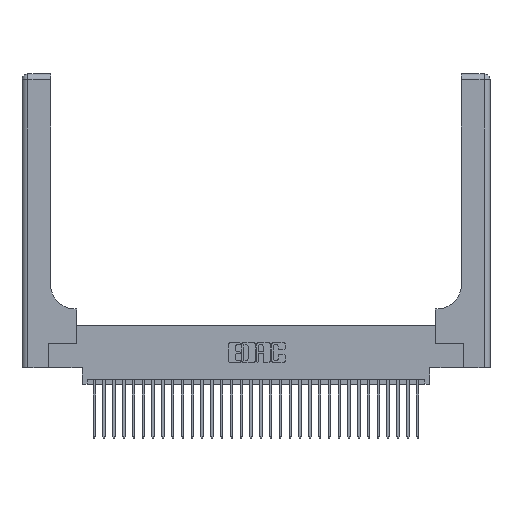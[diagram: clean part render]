
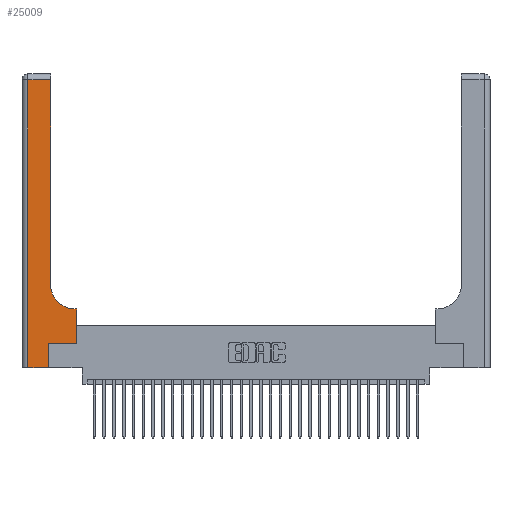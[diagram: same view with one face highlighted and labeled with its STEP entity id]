
A CAD part, top view. The second image highlights one B-rep face of the part: STEP entity #25009.
In plain terms, the highlighted planar face has unit normal (0, 0, 1).
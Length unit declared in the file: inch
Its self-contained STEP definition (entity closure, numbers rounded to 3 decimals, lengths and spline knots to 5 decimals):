
#437 = LINE ( 'NONE', #23626, #13341 ) ;
#452 = CARTESIAN_POINT ( 'NONE',  ( 0.2915, 3., 0.37 ) ) ;
#561 = CARTESIAN_POINT ( 'NONE',  ( 0.2915, 0.6, 0.37 ) ) ;
#865 = CARTESIAN_POINT ( 'NONE',  ( 0.2915, 2.94, 0.37 ) ) ;
#1384 = CARTESIAN_POINT ( 'NONE',  ( 0.269, 0., 0.37 ) ) ;
#1881 = VERTEX_POINT ( 'NONE', #16991 ) ;
#2483 = ORIENTED_EDGE ( 'NONE', *, *, #30789, .T. ) ;
#2496 = CARTESIAN_POINT ( 'NONE',  ( 0.2915, 0.85, 0.37 ) ) ;
#3045 = ORIENTED_EDGE ( 'NONE', *, *, #4793, .T. ) ;
#3761 = DIRECTION ( 'NONE',  ( 0., 1., 0. ) ) ;
#4261 = VECTOR ( 'NONE', #16527, 39.37008 ) ;
#4507 = AXIS2_PLACEMENT_3D ( 'NONE', #21239, #13704, #13822 ) ;
#4793 = EDGE_CURVE ( 'NONE', #21407, #13667, #21918, .T. ) ;
#5126 = LINE ( 'NONE', #13885, #5511 ) ;
#5150 = AXIS2_PLACEMENT_3D ( 'NONE', #10960, #29333, #16827 ) ;
#5359 = VERTEX_POINT ( 'NONE', #17052 ) ;
#5511 = VECTOR ( 'NONE', #26404, 39.37008 ) ;
#5769 = CARTESIAN_POINT ( 'NONE',  ( 0.5415, 0.6, 0.37 ) ) ;
#5824 = LINE ( 'NONE', #1384, #4261 ) ;
#6799 = EDGE_CURVE ( 'NONE', #12042, #1881, #5824, .T. ) ;
#7576 = LINE ( 'NONE', #21021, #11611 ) ;
#8176 = EDGE_CURVE ( 'NONE', #11689, #12443, #8550, .T. ) ;
#8550 = CIRCLE ( 'NONE', #4507, 0.25 ) ;
#9730 = CARTESIAN_POINT ( 'NONE',  ( 0.5585, 0.25, 0.37 ) ) ;
#9864 = ORIENTED_EDGE ( 'NONE', *, *, #23254, .T. ) ;
#10960 = CARTESIAN_POINT ( 'NONE',  ( 0., 3., 0.37 ) ) ;
#11039 = VERTEX_POINT ( 'NONE', #9730 ) ;
#11091 = FACE_OUTER_BOUND ( 'NONE', #13476, .T. ) ;
#11585 = CARTESIAN_POINT ( 'NONE',  ( 0.269, 0., 0.37 ) ) ;
#11611 = VECTOR ( 'NONE', #15913, 39.37008 ) ;
#11689 = VERTEX_POINT ( 'NONE', #5769 ) ;
#11744 = EDGE_CURVE ( 'NONE', #1881, #11039, #437, .T. ) ;
#11920 = LINE ( 'NONE', #22999, #21047 ) ;
#12042 = VERTEX_POINT ( 'NONE', #11585 ) ;
#12222 = LINE ( 'NONE', #452, #17028 ) ;
#12385 = VECTOR ( 'NONE', #31955, 39.37008 ) ;
#12443 = VERTEX_POINT ( 'NONE', #2496 ) ;
#13009 = ORIENTED_EDGE ( 'NONE', *, *, #11744, .T. ) ;
#13341 = VECTOR ( 'NONE', #16096, 39.37008 ) ;
#13438 = LINE ( 'NONE', #561, #26152 ) ;
#13476 = EDGE_LOOP ( 'NONE', ( #9864, #3045, #22827, #26286, #18869, #13009, #2483, #15066, #29389 ) ) ;
#13667 = VERTEX_POINT ( 'NONE', #14462 ) ;
#13704 = DIRECTION ( 'NONE',  ( 0., 0., -1. ) ) ;
#13822 = DIRECTION ( 'NONE',  ( 1., 0., 0. ) ) ;
#13885 = CARTESIAN_POINT ( 'NONE',  ( 0.5585, 0.25, 0.37 ) ) ;
#14462 = CARTESIAN_POINT ( 'NONE',  ( 0.06, 2.94, 0.37 ) ) ;
#15066 = ORIENTED_EDGE ( 'NONE', *, *, #22083, .T. ) ;
#15913 = DIRECTION ( 'NONE',  ( 1., 0., 0. ) ) ;
#16096 = DIRECTION ( 'NONE',  ( 1., 0., 0. ) ) ;
#16527 = DIRECTION ( 'NONE',  ( 0., 1., 0. ) ) ;
#16827 = DIRECTION ( 'NONE',  ( -1., 0., 0. ) ) ;
#16991 = CARTESIAN_POINT ( 'NONE',  ( 0.269, 0.25, 0.37 ) ) ;
#17028 = VECTOR ( 'NONE', #3761, 39.37008 ) ;
#17052 = CARTESIAN_POINT ( 'NONE',  ( 0.5585, 0.6, 0.37 ) ) ;
#18869 = ORIENTED_EDGE ( 'NONE', *, *, #6799, .T. ) ;
#18910 = VERTEX_POINT ( 'NONE', #25237 ) ;
#19452 = EDGE_CURVE ( 'NONE', #18910, #12042, #7576, .T. ) ;
#21021 = CARTESIAN_POINT ( 'NONE',  ( 0., 0., 0.37 ) ) ;
#21047 = VECTOR ( 'NONE', #30774, 39.37008 ) ;
#21239 = CARTESIAN_POINT ( 'NONE',  ( 0.5415, 0.85, 0.37 ) ) ;
#21407 = VERTEX_POINT ( 'NONE', #865 ) ;
#21918 = LINE ( 'NONE', #27706, #12385 ) ;
#22083 = EDGE_CURVE ( 'NONE', #5359, #11689, #13438, .T. ) ;
#22827 = ORIENTED_EDGE ( 'NONE', *, *, #31845, .T. ) ;
#22999 = CARTESIAN_POINT ( 'NONE',  ( 0.06, 3., 0.37 ) ) ;
#23254 = EDGE_CURVE ( 'NONE', #12443, #21407, #12222, .T. ) ;
#23626 = CARTESIAN_POINT ( 'NONE',  ( 0.269, 0.25, 0.37 ) ) ;
#25009 = ADVANCED_FACE ( 'NONE', ( #11091 ), #26235, .F. ) ;
#25237 = CARTESIAN_POINT ( 'NONE',  ( 0.06, 0., 0.37 ) ) ;
#26152 = VECTOR ( 'NONE', #28924, 39.37008 ) ;
#26235 = PLANE ( 'NONE',  #5150 ) ;
#26286 = ORIENTED_EDGE ( 'NONE', *, *, #19452, .T. ) ;
#26404 = DIRECTION ( 'NONE',  ( 0., 1., 0. ) ) ;
#27706 = CARTESIAN_POINT ( 'NONE',  ( 0., 2.94, 0.37 ) ) ;
#28924 = DIRECTION ( 'NONE',  ( -1., 0., 0. ) ) ;
#29333 = DIRECTION ( 'NONE',  ( 0., 0., -1. ) ) ;
#29389 = ORIENTED_EDGE ( 'NONE', *, *, #8176, .T. ) ;
#30774 = DIRECTION ( 'NONE',  ( 0., -1., 0. ) ) ;
#30789 = EDGE_CURVE ( 'NONE', #11039, #5359, #5126, .T. ) ;
#31845 = EDGE_CURVE ( 'NONE', #13667, #18910, #11920, .T. ) ;
#31955 = DIRECTION ( 'NONE',  ( -1., 0., 0. ) ) ;
